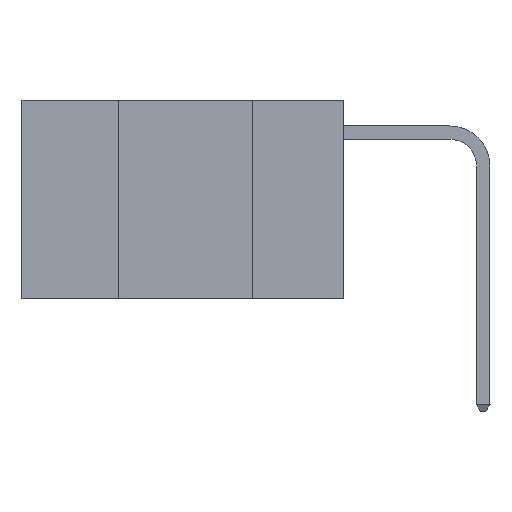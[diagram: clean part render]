
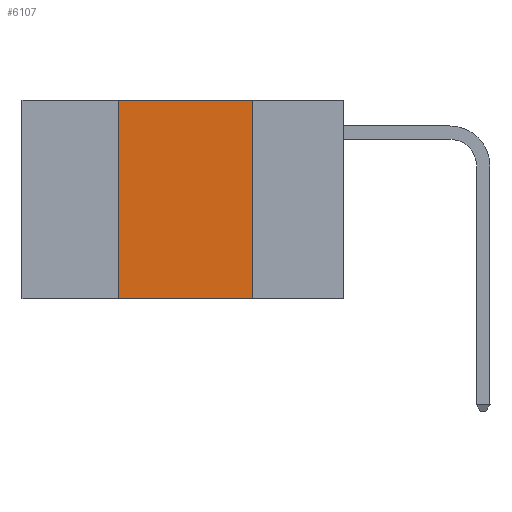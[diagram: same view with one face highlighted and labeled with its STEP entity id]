
A CAD part, left-side view. The second image highlights one B-rep face of the part: STEP entity #6107.
In plain terms, the highlighted planar face has unit normal (-1, 0, 0).
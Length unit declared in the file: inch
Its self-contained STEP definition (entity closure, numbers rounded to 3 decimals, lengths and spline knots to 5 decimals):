
#42 = CARTESIAN_POINT ( 'NONE',  ( 0., 0.6, -0.37 ) ) ;
#60 = AXIS2_PLACEMENT_3D ( 'NONE', #5498, #3534, #6813 ) ;
#71 = CARTESIAN_POINT ( 'NONE',  ( 0., 0.17, 0. ) ) ;
#277 = EDGE_LOOP ( 'NONE', ( #2207, #1366, #3872, #1302 ) ) ;
#735 = DIRECTION ( 'NONE',  ( 0., -1., 0. ) ) ;
#884 = VECTOR ( 'NONE', #735, 39.37008 ) ;
#1016 = VERTEX_POINT ( 'NONE', #3704 ) ;
#1083 = VECTOR ( 'NONE', #1253, 39.37008 ) ;
#1127 = EDGE_CURVE ( 'NONE', #6635, #7275, #7628, .T. ) ;
#1253 = DIRECTION ( 'NONE',  ( 0., 0., 1. ) ) ;
#1302 = ORIENTED_EDGE ( 'NONE', *, *, #6923, .T. ) ;
#1366 = ORIENTED_EDGE ( 'NONE', *, *, #5444, .F. ) ;
#1882 = DIRECTION ( 'NONE',  ( 0., 0., -1. ) ) ;
#2201 = EDGE_CURVE ( 'NONE', #1016, #7064, #7154, .T. ) ;
#2207 = ORIENTED_EDGE ( 'NONE', *, *, #2201, .F. ) ;
#3107 = CARTESIAN_POINT ( 'NONE',  ( 0., 0.42, -0.37 ) ) ;
#3534 = DIRECTION ( 'NONE',  ( 1., 0., 0. ) ) ;
#3704 = CARTESIAN_POINT ( 'NONE',  ( 0., 0.17, 0. ) ) ;
#3768 = DIRECTION ( 'NONE',  ( 0., -1., 0. ) ) ;
#3872 = ORIENTED_EDGE ( 'NONE', *, *, #1127, .F. ) ;
#4099 = CARTESIAN_POINT ( 'NONE',  ( 0., 0.17, -0.37 ) ) ;
#4161 = PLANE ( 'NONE',  #60 ) ;
#4432 = LINE ( 'NONE', #7487, #6359 ) ;
#4450 = CARTESIAN_POINT ( 'NONE',  ( 0., 0.42, 0. ) ) ;
#4988 = VECTOR ( 'NONE', #1882, 39.37008 ) ;
#5444 = EDGE_CURVE ( 'NONE', #7275, #1016, #4432, .T. ) ;
#5498 = CARTESIAN_POINT ( 'NONE',  ( 0., 0.6, 0. ) ) ;
#6107 = ADVANCED_FACE ( 'NONE', ( #7923 ), #4161, .F. ) ;
#6359 = VECTOR ( 'NONE', #3768, 39.37008 ) ;
#6474 = LINE ( 'NONE', #42, #884 ) ;
#6635 = VERTEX_POINT ( 'NONE', #3107 ) ;
#6813 = DIRECTION ( 'NONE',  ( 0., 0., -1. ) ) ;
#6923 = EDGE_CURVE ( 'NONE', #6635, #7064, #6474, .T. ) ;
#7064 = VERTEX_POINT ( 'NONE', #4099 ) ;
#7154 = LINE ( 'NONE', #71, #4988 ) ;
#7275 = VERTEX_POINT ( 'NONE', #8061 ) ;
#7487 = CARTESIAN_POINT ( 'NONE',  ( 0., 0.6, 0. ) ) ;
#7628 = LINE ( 'NONE', #4450, #1083 ) ;
#7923 = FACE_OUTER_BOUND ( 'NONE', #277, .T. ) ;
#8061 = CARTESIAN_POINT ( 'NONE',  ( 0., 0.42, 0. ) ) ;
